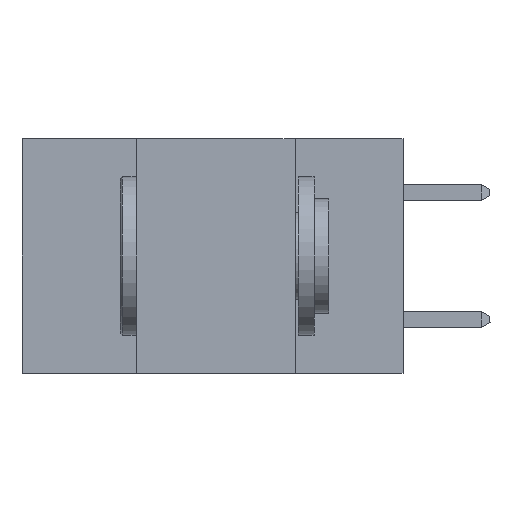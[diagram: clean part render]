
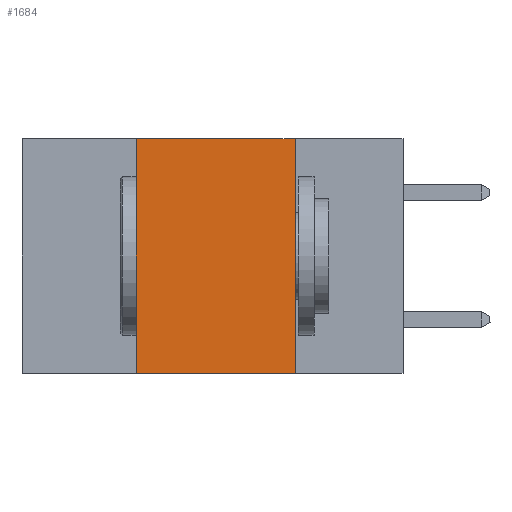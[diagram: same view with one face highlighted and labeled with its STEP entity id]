
A CAD part, left-side view. The second image highlights one B-rep face of the part: STEP entity #1684.
In plain terms, the highlighted planar face has unit normal (-1, 0, 0).
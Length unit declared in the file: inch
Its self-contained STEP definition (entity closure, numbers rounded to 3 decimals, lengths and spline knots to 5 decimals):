
#60 = FACE_OUTER_BOUND ( 'NONE', #12254, .T. ) ;
#1684 = ADVANCED_FACE ( 'NONE', ( #60 ), #6496, .F. ) ;
#1706 = CARTESIAN_POINT ( 'NONE',  ( 0., 0.6, 0. ) ) ;
#2279 = DIRECTION ( 'NONE',  ( 1., 0., 0. ) ) ;
#2791 = VECTOR ( 'NONE', #3482, 39.37008 ) ;
#3482 = DIRECTION ( 'NONE',  ( 0., 0., -1. ) ) ;
#4688 = ORIENTED_EDGE ( 'NONE', *, *, #6351, .F. ) ;
#5283 = VERTEX_POINT ( 'NONE', #15003 ) ;
#5689 = AXIS2_PLACEMENT_3D ( 'NONE', #10993, #2279, #9395 ) ;
#5748 = EDGE_CURVE ( 'NONE', #8508, #5283, #14679, .T. ) ;
#5859 = EDGE_CURVE ( 'NONE', #5283, #16791, #12209, .T. ) ;
#5971 = VECTOR ( 'NONE', #9359, 39.37008 ) ;
#6351 = EDGE_CURVE ( 'NONE', #16791, #12970, #8549, .T. ) ;
#6496 = PLANE ( 'NONE',  #5689 ) ;
#7304 = CARTESIAN_POINT ( 'NONE',  ( 0., 0.17, 0. ) ) ;
#7501 = CARTESIAN_POINT ( 'NONE',  ( 0., 0.42, -0.37 ) ) ;
#8119 = CARTESIAN_POINT ( 'NONE',  ( 0., 0.17, -0.37 ) ) ;
#8314 = ORIENTED_EDGE ( 'NONE', *, *, #5859, .F. ) ;
#8336 = VECTOR ( 'NONE', #10364, 39.37008 ) ;
#8508 = VERTEX_POINT ( 'NONE', #7501 ) ;
#8549 = LINE ( 'NONE', #12292, #2791 ) ;
#9089 = CARTESIAN_POINT ( 'NONE',  ( 0., 0.42, 0. ) ) ;
#9359 = DIRECTION ( 'NONE',  ( 0., -1., 0. ) ) ;
#9395 = DIRECTION ( 'NONE',  ( 0., 0., -1. ) ) ;
#9504 = DIRECTION ( 'NONE',  ( 0., -1., 0. ) ) ;
#10364 = DIRECTION ( 'NONE',  ( 0., 0., 1. ) ) ;
#10993 = CARTESIAN_POINT ( 'NONE',  ( 0., 0.6, 0. ) ) ;
#11420 = ORIENTED_EDGE ( 'NONE', *, *, #5748, .F. ) ;
#11440 = EDGE_CURVE ( 'NONE', #8508, #12970, #14178, .T. ) ;
#11751 = VECTOR ( 'NONE', #9504, 39.37008 ) ;
#12209 = LINE ( 'NONE', #1706, #11751 ) ;
#12254 = EDGE_LOOP ( 'NONE', ( #4688, #8314, #11420, #18318 ) ) ;
#12292 = CARTESIAN_POINT ( 'NONE',  ( 0., 0.17, 0. ) ) ;
#12970 = VERTEX_POINT ( 'NONE', #8119 ) ;
#14178 = LINE ( 'NONE', #18014, #5971 ) ;
#14679 = LINE ( 'NONE', #9089, #8336 ) ;
#15003 = CARTESIAN_POINT ( 'NONE',  ( 0., 0.42, 0. ) ) ;
#16791 = VERTEX_POINT ( 'NONE', #7304 ) ;
#18014 = CARTESIAN_POINT ( 'NONE',  ( 0., 0.6, -0.37 ) ) ;
#18318 = ORIENTED_EDGE ( 'NONE', *, *, #11440, .T. ) ;
